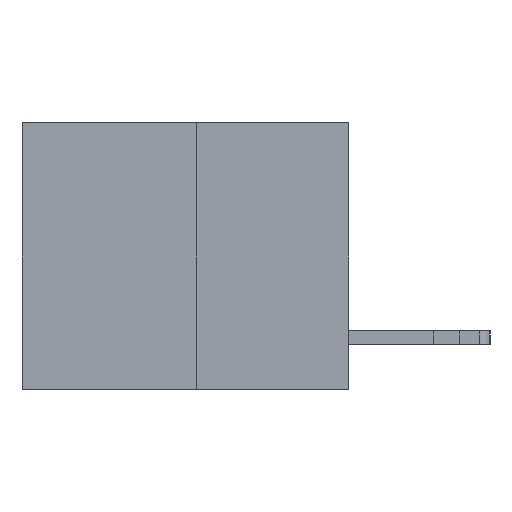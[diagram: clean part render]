
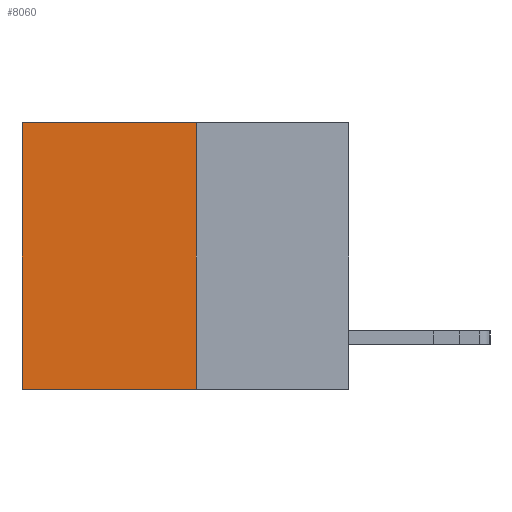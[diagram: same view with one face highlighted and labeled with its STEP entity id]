
A CAD part, left-side view. The second image highlights one B-rep face of the part: STEP entity #8060.
In plain terms, the highlighted planar face has unit normal (-1, 0, 0).
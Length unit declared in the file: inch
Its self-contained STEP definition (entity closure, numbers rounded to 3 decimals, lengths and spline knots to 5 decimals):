
#1803 = ORIENTED_EDGE ( 'NONE', *, *, #14377, .T. ) ;
#1834 = CARTESIAN_POINT ( 'NONE',  ( 0.3165, 0.28, 0. ) ) ;
#2112 = VERTEX_POINT ( 'NONE', #1834 ) ;
#2166 = PLANE ( 'NONE',  #14427 ) ;
#2279 = CARTESIAN_POINT ( 'NONE',  ( 0.3165, 0.28, 0. ) ) ;
#2759 = LINE ( 'NONE', #6240, #5489 ) ;
#2791 = CARTESIAN_POINT ( 'NONE',  ( 0.3165, 0.6, 0. ) ) ;
#3263 = FACE_OUTER_BOUND ( 'NONE', #3593, .T. ) ;
#3593 = EDGE_LOOP ( 'NONE', ( #1803, #10159, #10819, #8524 ) ) ;
#3660 = DIRECTION ( 'NONE',  ( 0., 0., -1. ) ) ;
#4008 = DIRECTION ( 'NONE',  ( 0., 0., -1. ) ) ;
#4711 = VECTOR ( 'NONE', #3660, 39.37008 ) ;
#5166 = VERTEX_POINT ( 'NONE', #2791 ) ;
#5489 = VECTOR ( 'NONE', #4008, 39.37008 ) ;
#5564 = CARTESIAN_POINT ( 'NONE',  ( 0.3165, 0.28, -0.49 ) ) ;
#5728 = CARTESIAN_POINT ( 'NONE',  ( 0.3165, 0.28, -0.49 ) ) ;
#5741 = CARTESIAN_POINT ( 'NONE',  ( 0.3165, 0.6, -0.49 ) ) ;
#6064 = VECTOR ( 'NONE', #14967, 39.37008 ) ;
#6240 = CARTESIAN_POINT ( 'NONE',  ( 0.3165, 0.6, -0.49 ) ) ;
#7079 = VERTEX_POINT ( 'NONE', #5741 ) ;
#7236 = CARTESIAN_POINT ( 'NONE',  ( 0.3165, 0.28, -0.49 ) ) ;
#7932 = EDGE_CURVE ( 'NONE', #2112, #5166, #10170, .T. ) ;
#8060 = ADVANCED_FACE ( 'NONE', ( #3263 ), #2166, .F. ) ;
#8400 = EDGE_CURVE ( 'NONE', #2112, #9403, #13954, .T. ) ;
#8524 = ORIENTED_EDGE ( 'NONE', *, *, #7932, .T. ) ;
#9156 = DIRECTION ( 'NONE',  ( 0., 0., -1. ) ) ;
#9403 = VERTEX_POINT ( 'NONE', #5728 ) ;
#9867 = LINE ( 'NONE', #14235, #6064 ) ;
#10159 = ORIENTED_EDGE ( 'NONE', *, *, #12090, .F. ) ;
#10170 = LINE ( 'NONE', #2279, #10531 ) ;
#10531 = VECTOR ( 'NONE', #12622, 39.37008 ) ;
#10819 = ORIENTED_EDGE ( 'NONE', *, *, #8400, .F. ) ;
#11445 = DIRECTION ( 'NONE',  ( 1., 0., 0. ) ) ;
#12090 = EDGE_CURVE ( 'NONE', #9403, #7079, #9867, .T. ) ;
#12622 = DIRECTION ( 'NONE',  ( 0., 1., 0. ) ) ;
#13954 = LINE ( 'NONE', #7236, #4711 ) ;
#14235 = CARTESIAN_POINT ( 'NONE',  ( 0.3165, 0.28, -0.49 ) ) ;
#14377 = EDGE_CURVE ( 'NONE', #5166, #7079, #2759, .T. ) ;
#14427 = AXIS2_PLACEMENT_3D ( 'NONE', #5564, #11445, #9156 ) ;
#14967 = DIRECTION ( 'NONE',  ( 0., 1., 0. ) ) ;
